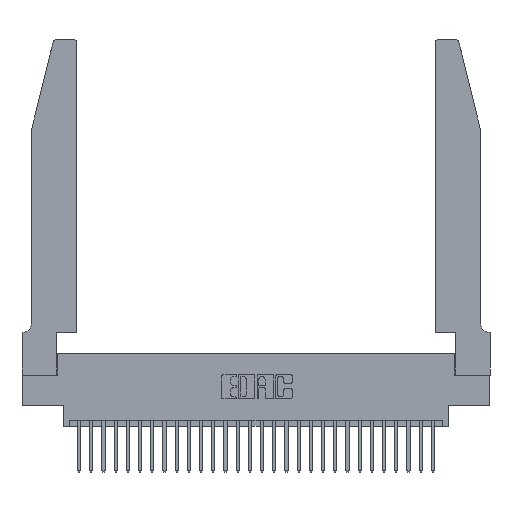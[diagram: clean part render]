
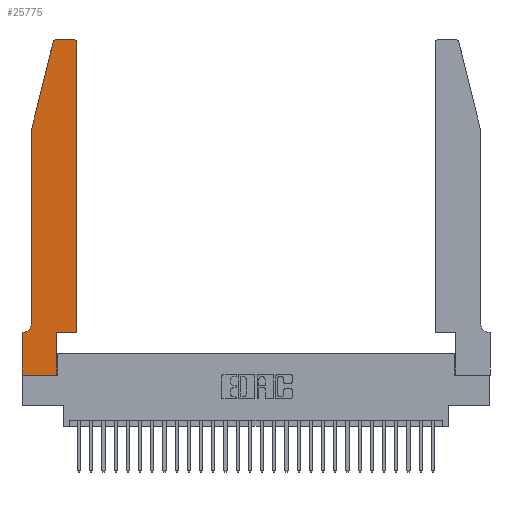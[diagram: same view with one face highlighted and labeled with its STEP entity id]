
A CAD part, top view. The second image highlights one B-rep face of the part: STEP entity #25775.
In plain terms, the highlighted planar face has unit normal (0, 0, 1).
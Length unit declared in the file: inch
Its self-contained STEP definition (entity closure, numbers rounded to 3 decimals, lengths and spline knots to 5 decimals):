
#847 = ORIENTED_EDGE ( 'NONE', *, *, #29106, .T. ) ;
#1395 = EDGE_CURVE ( 'NONE', #3137, #14926, #13858, .T. ) ;
#1771 = CARTESIAN_POINT ( 'NONE',  ( 0.4505, 0.35, 0.37 ) ) ;
#1813 = VERTEX_POINT ( 'NONE', #14319 ) ;
#1883 = VECTOR ( 'NONE', #15911, 39.37008 ) ;
#2066 = DIRECTION ( 'NONE',  ( -1., 0., 0. ) ) ;
#2485 = CARTESIAN_POINT ( 'NONE',  ( 0., 0., 0.37 ) ) ;
#2617 = EDGE_CURVE ( 'NONE', #14926, #12813, #22181, .T. ) ;
#2618 = VERTEX_POINT ( 'NONE', #9890 ) ;
#3077 = ORIENTED_EDGE ( 'NONE', *, *, #13021, .T. ) ;
#3137 = VERTEX_POINT ( 'NONE', #1771 ) ;
#3789 = CARTESIAN_POINT ( 'NONE',  ( 0.0755, 2., 0.37 ) ) ;
#4258 = VERTEX_POINT ( 'NONE', #15639 ) ;
#4596 = CARTESIAN_POINT ( 'NONE',  ( 0.284, 2.75, 0.37 ) ) ;
#4740 = EDGE_CURVE ( 'NONE', #21062, #2618, #28477, .T. ) ;
#4896 = VECTOR ( 'NONE', #13172, 39.37008 ) ;
#5006 = AXIS2_PLACEMENT_3D ( 'NONE', #22158, #8309, #24442 ) ;
#6036 = CIRCLE ( 'NONE', #30013, 0.07 ) ;
#6339 = FACE_OUTER_BOUND ( 'NONE', #11683, .T. ) ;
#6591 = CARTESIAN_POINT ( 'NONE',  ( 0.4505, 0.35, 0.37 ) ) ;
#8148 = LINE ( 'NONE', #20349, #25087 ) ;
#8309 = DIRECTION ( 'NONE',  ( 0., 0., 1. ) ) ;
#9676 = PLANE ( 'NONE',  #15080 ) ;
#9890 = CARTESIAN_POINT ( 'NONE',  ( 0.25487, 2.72718, 0.37 ) ) ;
#10400 = DIRECTION ( 'NONE',  ( 0., 1., 0. ) ) ;
#10469 = EDGE_CURVE ( 'NONE', #2618, #27139, #20963, .T. ) ;
#11158 = ORIENTED_EDGE ( 'NONE', *, *, #17068, .T. ) ;
#11391 = DIRECTION ( 'NONE',  ( 0., 1., 0. ) ) ;
#11432 = CARTESIAN_POINT ( 'NONE',  ( 0.2605, 2.75, 0.37 ) ) ;
#11683 = EDGE_LOOP ( 'NONE', ( #15435, #18332, #20485, #25494, #23713, #12598, #3077, #11158, #847, #25935, #15191, #24785 ) ) ;
#11929 = CARTESIAN_POINT ( 'NONE',  ( 0., 0.35, 0.37 ) ) ;
#12016 = DIRECTION ( 'NONE',  ( 1., 0., 0. ) ) ;
#12598 = ORIENTED_EDGE ( 'NONE', *, *, #29820, .T. ) ;
#12611 = CARTESIAN_POINT ( 'NONE',  ( 0.4205, 2.72, 0.37 ) ) ;
#12670 = CARTESIAN_POINT ( 'NONE',  ( 0.0055, 0.42, 0.37 ) ) ;
#12763 = AXIS2_PLACEMENT_3D ( 'NONE', #12611, #17416, #16435 ) ;
#12813 = VERTEX_POINT ( 'NONE', #12818 ) ;
#12818 = CARTESIAN_POINT ( 'NONE',  ( 0.4205, 2.75, 0.37 ) ) ;
#13021 = EDGE_CURVE ( 'NONE', #4258, #23378, #8148, .T. ) ;
#13172 = DIRECTION ( 'NONE',  ( 0., -1., 0. ) ) ;
#13577 = EDGE_CURVE ( 'NONE', #27139, #22396, #29380, .T. ) ;
#13755 = EDGE_CURVE ( 'NONE', #12813, #21062, #19032, .T. ) ;
#13858 = LINE ( 'NONE', #6591, #25348 ) ;
#14182 = VERTEX_POINT ( 'NONE', #17483 ) ;
#14319 = CARTESIAN_POINT ( 'NONE',  ( 0.2865, 0., 0.37 ) ) ;
#14355 = LINE ( 'NONE', #22750, #1883 ) ;
#14869 = VECTOR ( 'NONE', #24607, 39.37008 ) ;
#14926 = VERTEX_POINT ( 'NONE', #22532 ) ;
#14986 = DIRECTION ( 'NONE',  ( -1., 0., 0. ) ) ;
#15080 = AXIS2_PLACEMENT_3D ( 'NONE', #11929, #25785, #12016 ) ;
#15191 = ORIENTED_EDGE ( 'NONE', *, *, #1395, .T. ) ;
#15435 = ORIENTED_EDGE ( 'NONE', *, *, #13755, .T. ) ;
#15442 = CARTESIAN_POINT ( 'NONE',  ( 0.0755, 2., 0.37 ) ) ;
#15538 = LINE ( 'NONE', #2485, #20926 ) ;
#15639 = CARTESIAN_POINT ( 'NONE',  ( 0., 0.35, 0.37 ) ) ;
#15911 = DIRECTION ( 'NONE',  ( -1., 0., 0. ) ) ;
#16435 = DIRECTION ( 'NONE',  ( 1., 0., 0. ) ) ;
#16799 = CARTESIAN_POINT ( 'NONE',  ( 0.0755, 0.42, 0.37 ) ) ;
#17068 = EDGE_CURVE ( 'NONE', #23378, #1813, #15538, .T. ) ;
#17416 = DIRECTION ( 'NONE',  ( 0., 0., 1. ) ) ;
#17483 = CARTESIAN_POINT ( 'NONE',  ( 0.2865, 0.35, 0.37 ) ) ;
#18149 = LINE ( 'NONE', #20270, #29576 ) ;
#18310 = VECTOR ( 'NONE', #2066, 39.37008 ) ;
#18332 = ORIENTED_EDGE ( 'NONE', *, *, #4740, .T. ) ;
#18732 = CARTESIAN_POINT ( 'NONE',  ( 0., 0., 0.37 ) ) ;
#19032 = LINE ( 'NONE', #11432, #18310 ) ;
#19333 = CARTESIAN_POINT ( 'NONE',  ( 0.0055, 0.35, 0.37 ) ) ;
#20270 = CARTESIAN_POINT ( 'NONE',  ( 0.4505, 0.35, 0.37 ) ) ;
#20349 = CARTESIAN_POINT ( 'NONE',  ( 0., 0., 0.37 ) ) ;
#20485 = ORIENTED_EDGE ( 'NONE', *, *, #10469, .T. ) ;
#20660 = VERTEX_POINT ( 'NONE', #19333 ) ;
#20926 = VECTOR ( 'NONE', #23409, 39.37008 ) ;
#20963 = LINE ( 'NONE', #3789, #14869 ) ;
#21062 = VERTEX_POINT ( 'NONE', #4596 ) ;
#21624 = VECTOR ( 'NONE', #10400, 39.37008 ) ;
#21652 = EDGE_CURVE ( 'NONE', #14182, #3137, #18149, .T. ) ;
#22158 = CARTESIAN_POINT ( 'NONE',  ( 0.284, 2.72, 0.37 ) ) ;
#22181 = CIRCLE ( 'NONE', #12763, 0.03 ) ;
#22396 = VERTEX_POINT ( 'NONE', #16799 ) ;
#22532 = CARTESIAN_POINT ( 'NONE',  ( 0.4505, 2.72, 0.37 ) ) ;
#22569 = DIRECTION ( 'NONE',  ( 1., 0., 0. ) ) ;
#22750 = CARTESIAN_POINT ( 'NONE',  ( 0.0755, 0.35, 0.37 ) ) ;
#23378 = VERTEX_POINT ( 'NONE', #18732 ) ;
#23409 = DIRECTION ( 'NONE',  ( 1., 0., 0. ) ) ;
#23713 = ORIENTED_EDGE ( 'NONE', *, *, #25299, .T. ) ;
#24442 = DIRECTION ( 'NONE',  ( 1., 0., 0. ) ) ;
#24603 = CARTESIAN_POINT ( 'NONE',  ( 0.0755, 2., 0.37 ) ) ;
#24607 = DIRECTION ( 'NONE',  ( -0.239, -0.971, 0. ) ) ;
#24785 = ORIENTED_EDGE ( 'NONE', *, *, #2617, .T. ) ;
#24931 = DIRECTION ( 'NONE',  ( 0., -1., 0. ) ) ;
#25087 = VECTOR ( 'NONE', #24931, 39.37008 ) ;
#25299 = EDGE_CURVE ( 'NONE', #22396, #20660, #6036, .T. ) ;
#25348 = VECTOR ( 'NONE', #11391, 39.37008 ) ;
#25494 = ORIENTED_EDGE ( 'NONE', *, *, #13577, .T. ) ;
#25775 = ADVANCED_FACE ( 'NONE', ( #6339 ), #9676, .T. ) ;
#25785 = DIRECTION ( 'NONE',  ( 0., 0., 1. ) ) ;
#25935 = ORIENTED_EDGE ( 'NONE', *, *, #21652, .T. ) ;
#27139 = VERTEX_POINT ( 'NONE', #15442 ) ;
#27685 = LINE ( 'NONE', #28784, #21624 ) ;
#28477 = CIRCLE ( 'NONE', #5006, 0.03 ) ;
#28710 = DIRECTION ( 'NONE',  ( 0., 0., -1. ) ) ;
#28784 = CARTESIAN_POINT ( 'NONE',  ( 0.2865, 0.35, 0.37 ) ) ;
#29106 = EDGE_CURVE ( 'NONE', #1813, #14182, #27685, .T. ) ;
#29380 = LINE ( 'NONE', #24603, #4896 ) ;
#29576 = VECTOR ( 'NONE', #22569, 39.37008 ) ;
#29820 = EDGE_CURVE ( 'NONE', #20660, #4258, #14355, .T. ) ;
#30013 = AXIS2_PLACEMENT_3D ( 'NONE', #12670, #28710, #14986 ) ;
